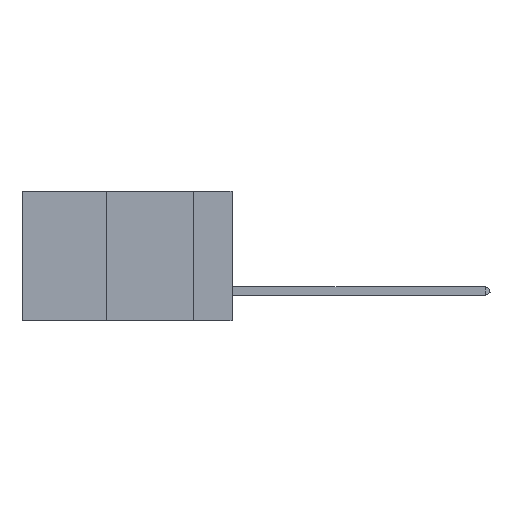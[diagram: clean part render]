
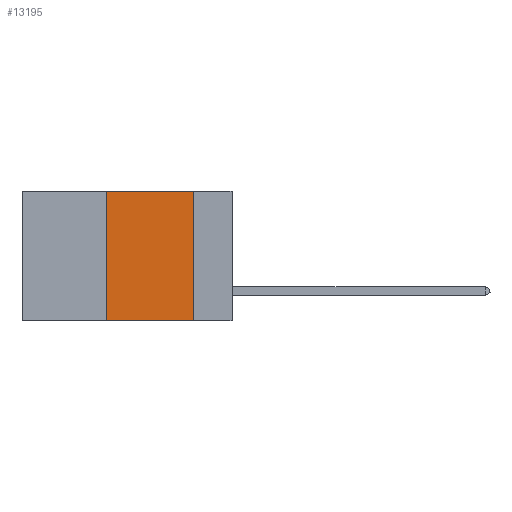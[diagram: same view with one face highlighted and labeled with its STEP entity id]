
A CAD part, left-side view. The second image highlights one B-rep face of the part: STEP entity #13195.
In plain terms, the highlighted planar face has unit normal (-1, 0, 0).
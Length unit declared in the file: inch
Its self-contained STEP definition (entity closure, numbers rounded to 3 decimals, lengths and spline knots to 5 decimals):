
#486 = DIRECTION ( 'NONE',  ( 0., -1., 0. ) ) ;
#868 = CARTESIAN_POINT ( 'NONE',  ( 0., 0.6, -0.37 ) ) ;
#2618 = LINE ( 'NONE', #6149, #14528 ) ;
#3135 = ORIENTED_EDGE ( 'NONE', *, *, #23361, .F. ) ;
#3576 = VERTEX_POINT ( 'NONE', #18601 ) ;
#4643 = VERTEX_POINT ( 'NONE', #18584 ) ;
#4786 = VERTEX_POINT ( 'NONE', #10982 ) ;
#5575 = ORIENTED_EDGE ( 'NONE', *, *, #19050, .T. ) ;
#5975 = EDGE_CURVE ( 'NONE', #4643, #3576, #23915, .T. ) ;
#6149 = CARTESIAN_POINT ( 'NONE',  ( 0., 0.11, 0. ) ) ;
#7573 = CARTESIAN_POINT ( 'NONE',  ( 0., 0.11, 0. ) ) ;
#9172 = LINE ( 'NONE', #23581, #15127 ) ;
#9870 = ORIENTED_EDGE ( 'NONE', *, *, #23892, .F. ) ;
#10982 = CARTESIAN_POINT ( 'NONE',  ( 0., 0.11, -0.37 ) ) ;
#11701 = AXIS2_PLACEMENT_3D ( 'NONE', #23199, #15718, #23030 ) ;
#12549 = FACE_OUTER_BOUND ( 'NONE', #18767, .T. ) ;
#13195 = ADVANCED_FACE ( 'NONE', ( #12549 ), #18821, .F. ) ;
#14008 = CARTESIAN_POINT ( 'NONE',  ( 0., 0.36, 0. ) ) ;
#14528 = VECTOR ( 'NONE', #15511, 39.37008 ) ;
#14658 = VERTEX_POINT ( 'NONE', #7573 ) ;
#15127 = VECTOR ( 'NONE', #486, 39.37008 ) ;
#15511 = DIRECTION ( 'NONE',  ( 0., 0., -1. ) ) ;
#15718 = DIRECTION ( 'NONE',  ( 1., 0., 0. ) ) ;
#17409 = VECTOR ( 'NONE', #19672, 39.37008 ) ;
#18584 = CARTESIAN_POINT ( 'NONE',  ( 0., 0.36, -0.37 ) ) ;
#18601 = CARTESIAN_POINT ( 'NONE',  ( 0., 0.36, 0. ) ) ;
#18767 = EDGE_LOOP ( 'NONE', ( #3135, #9870, #20049, #5575 ) ) ;
#18821 = PLANE ( 'NONE',  #11701 ) ;
#19050 = EDGE_CURVE ( 'NONE', #4643, #4786, #20995, .T. ) ;
#19672 = DIRECTION ( 'NONE',  ( 0., -1., 0. ) ) ;
#20049 = ORIENTED_EDGE ( 'NONE', *, *, #5975, .F. ) ;
#20589 = DIRECTION ( 'NONE',  ( 0., 0., 1. ) ) ;
#20907 = VECTOR ( 'NONE', #20589, 39.37008 ) ;
#20995 = LINE ( 'NONE', #868, #17409 ) ;
#23030 = DIRECTION ( 'NONE',  ( 0., 0., -1. ) ) ;
#23199 = CARTESIAN_POINT ( 'NONE',  ( 0., 0.6, 0. ) ) ;
#23361 = EDGE_CURVE ( 'NONE', #14658, #4786, #2618, .T. ) ;
#23581 = CARTESIAN_POINT ( 'NONE',  ( 0., 0.6, 0. ) ) ;
#23892 = EDGE_CURVE ( 'NONE', #3576, #14658, #9172, .T. ) ;
#23915 = LINE ( 'NONE', #14008, #20907 ) ;
